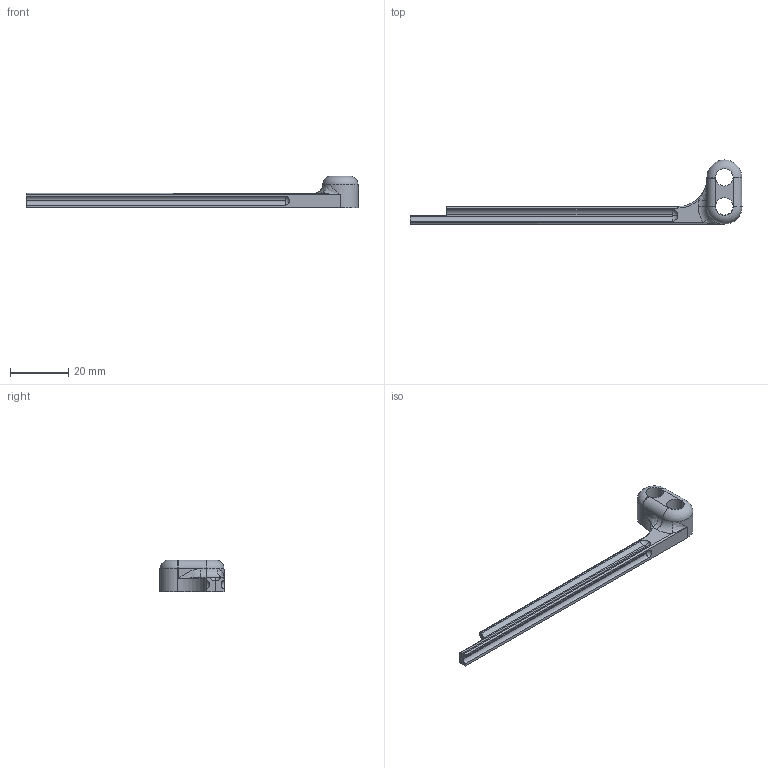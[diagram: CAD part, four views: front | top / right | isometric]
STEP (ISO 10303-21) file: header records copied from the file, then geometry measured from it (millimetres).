
FILE_DESCRIPTION (( 'STEP AP214' ), '1' );
FILE_NAME ('Trigger_Rod_Left_1.step', '2014-05-14T06:09:44', ( 'WarFairy' ), ( '' ), 'SwSTEP 2.0', 'SolidWorks 2013', '' );
FILE_SCHEMA (( 'AUTOMOTIVE_DESIGN' ));
Length unit declared in the file: inch
Products named in the file (1): Trigger_Rod_Left_1
Bounding box: 114.3 x 22.07 x 11 mm (x, y, z)
Volume: 4261.2 mm3; surface area: 3684.4 mm2
Topology: 1 solids, 1 shells, 48 faces, 123 edges, 75 vertices
Faces by surface type: cylinder 20, plane 14, torus 12, bspline 2
Entity records: 1811 total; most frequent: CARTESIAN_POINT 594, DIRECTION 257, ORIENTED_EDGE 244, EDGE_CURVE 122, AXIS2_PLACEMENT_3D 100, VERTEX_POINT 75, VECTOR 57, LINE 57
